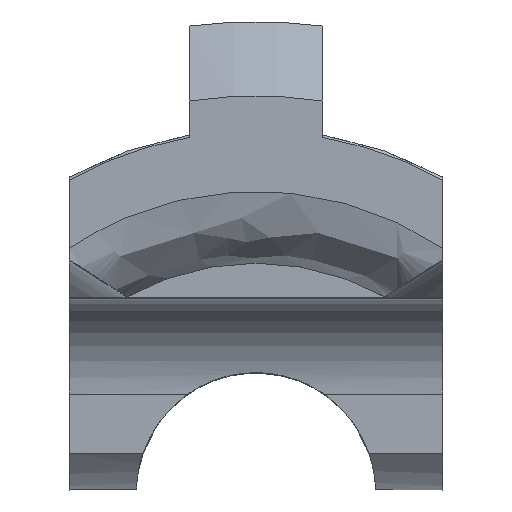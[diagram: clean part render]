
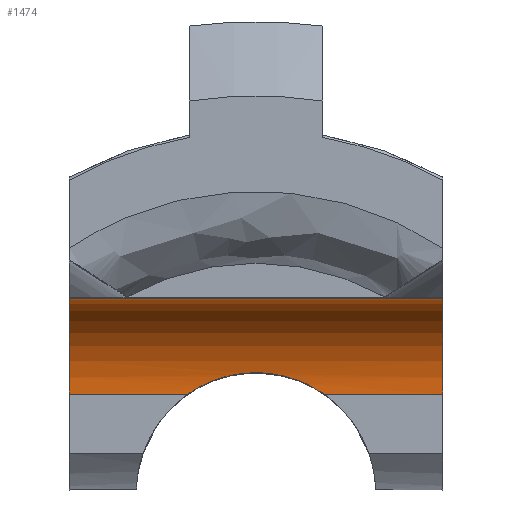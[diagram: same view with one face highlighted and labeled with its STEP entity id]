
A CAD part, top view. The second image highlights one B-rep face of the part: STEP entity #1474.
In plain terms, the highlighted cylindrical face has radius 1.587 mm (diameter 3.175 mm), a partial arc.
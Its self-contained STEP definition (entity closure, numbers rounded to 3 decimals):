
#36 = EDGE_LOOP ( 'NONE', ( #790, #792, #795, #941, #957, #829 ) ) ;
#103 = CARTESIAN_POINT ( 'NONE',  ( 3.099, -0.762, 4.28 ) ) ;
#162 = LINE ( 'NONE', #827, #336 ) ;
#195 = AXIS2_PLACEMENT_3D ( 'NONE', #1068, #1304, #1166 ) ;
#263 = VERTEX_POINT ( 'NONE', #755 ) ;
#272 = AXIS2_PLACEMENT_3D ( 'NONE', #103, #1405, #918 ) ;
#298 = EDGE_CURVE ( 'NONE', #670, #1162, #162, .T. ) ;
#308 = EDGE_CURVE ( 'NONE', #1499, #1197, #1415, .T. ) ;
#334 = EDGE_CURVE ( 'NONE', #1162, #1499, #448, .T. ) ;
#336 = VECTOR ( 'NONE', #819, 1000. ) ;
#375 = FACE_OUTER_BOUND ( 'NONE', #36, .T. ) ;
#448 = B_SPLINE_CURVE_WITH_KNOTS ( 'NONE', 3,
 ( #653, #704, #684, #648, #640, #637, #607, #587, #582, #569 ),
 .UNSPECIFIED., .F., .F.,
 ( 4, 2, 2, 2, 4 ),
 ( 0., 0.001, 0.001, 0.002, 0.002 ),
 .UNSPECIFIED. ) ;
#462 = VERTEX_POINT ( 'NONE', #698 ) ;
#569 = CARTESIAN_POINT ( 'NONE',  ( -1.134, -0.762, 2.692 ) ) ;
#582 = CARTESIAN_POINT ( 'NONE',  ( -0.967, -0.646, 2.692 ) ) ;
#587 = CARTESIAN_POINT ( 'NONE',  ( -0.783, -0.557, 2.705 ) ) ;
#607 = CARTESIAN_POINT ( 'NONE',  ( -0.401, -0.437, 2.725 ) ) ;
#618 = LINE ( 'NONE', #1178, #822 ) ;
#630 = VECTOR ( 'NONE', #785, 1000. ) ;
#637 = CARTESIAN_POINT ( 'NONE',  ( -0.199, -0.406, 2.733 ) ) ;
#640 = CARTESIAN_POINT ( 'NONE',  ( 0.203, -0.407, 2.733 ) ) ;
#641 = CARTESIAN_POINT ( 'NONE',  ( 3.099, -0.762, 4.28 ) ) ;
#648 = CARTESIAN_POINT ( 'NONE',  ( 0.403, -0.437, 2.725 ) ) ;
#653 = CARTESIAN_POINT ( 'NONE',  ( 1.134, -0.762, 2.692 ) ) ;
#664 = CARTESIAN_POINT ( 'NONE',  ( 1.134, -0.762, 2.692 ) ) ;
#669 = CARTESIAN_POINT ( 'NONE',  ( -3.099, -0.762, 2.692 ) ) ;
#670 = VERTEX_POINT ( 'NONE', #1289 ) ;
#684 = CARTESIAN_POINT ( 'NONE',  ( 0.787, -0.558, 2.704 ) ) ;
#698 = CARTESIAN_POINT ( 'NONE',  ( 3.099, 0.825, 4.28 ) ) ;
#704 = CARTESIAN_POINT ( 'NONE',  ( 0.967, -0.646, 2.692 ) ) ;
#749 = DIRECTION ( 'NONE',  ( -1., 0., 0. ) ) ;
#755 = CARTESIAN_POINT ( 'NONE',  ( -3.099, 0.825, 4.28 ) ) ;
#771 = CARTESIAN_POINT ( 'NONE',  ( 3.099, -0.762, 2.692 ) ) ;
#781 = CIRCLE ( 'NONE', #195, 1.588 ) ;
#785 = DIRECTION ( 'NONE',  ( -1., 0., 0. ) ) ;
#790 = ORIENTED_EDGE ( 'NONE', *, *, #334, .F. ) ;
#792 = ORIENTED_EDGE ( 'NONE', *, *, #298, .F. ) ;
#795 = ORIENTED_EDGE ( 'NONE', *, *, #884, .F. ) ;
#819 = DIRECTION ( 'NONE',  ( -1., 0., 0. ) ) ;
#822 = VECTOR ( 'NONE', #942, 1000. ) ;
#827 = CARTESIAN_POINT ( 'NONE',  ( 3.099, -0.762, 2.692 ) ) ;
#829 = ORIENTED_EDGE ( 'NONE', *, *, #308, .F. ) ;
#872 = EDGE_CURVE ( 'NONE', #263, #462, #618, .T. ) ;
#884 = EDGE_CURVE ( 'NONE', #462, #670, #1437, .T. ) ;
#905 = EDGE_CURVE ( 'NONE', #263, #1197, #781, .T. ) ;
#918 = DIRECTION ( 'NONE',  ( 0., 0., 1. ) ) ;
#941 = ORIENTED_EDGE ( 'NONE', *, *, #872, .F. ) ;
#942 = DIRECTION ( 'NONE',  ( 1., 0., 0. ) ) ;
#957 = ORIENTED_EDGE ( 'NONE', *, *, #905, .T. ) ;
#1006 = CARTESIAN_POINT ( 'NONE',  ( -1.134, -0.762, 2.692 ) ) ;
#1068 = CARTESIAN_POINT ( 'NONE',  ( -3.099, -0.762, 4.28 ) ) ;
#1162 = VERTEX_POINT ( 'NONE', #664 ) ;
#1166 = DIRECTION ( 'NONE',  ( 0., 0., 1. ) ) ;
#1178 = CARTESIAN_POINT ( 'NONE',  ( 3.099, 0.825, 4.28 ) ) ;
#1197 = VERTEX_POINT ( 'NONE', #669 ) ;
#1234 = CYLINDRICAL_SURFACE ( 'NONE', #1465, 1.588 ) ;
#1289 = CARTESIAN_POINT ( 'NONE',  ( 3.099, -0.762, 2.692 ) ) ;
#1304 = DIRECTION ( 'NONE',  ( -1., 0., 0. ) ) ;
#1361 = DIRECTION ( 'NONE',  ( 0., 0., 1. ) ) ;
#1405 = DIRECTION ( 'NONE',  ( -1., 0., 0. ) ) ;
#1415 = LINE ( 'NONE', #771, #630 ) ;
#1437 = CIRCLE ( 'NONE', #272, 1.588 ) ;
#1465 = AXIS2_PLACEMENT_3D ( 'NONE', #641, #749, #1361 ) ;
#1474 = ADVANCED_FACE ( 'NONE', ( #375 ), #1234, .F. ) ;
#1499 = VERTEX_POINT ( 'NONE', #1006 ) ;
